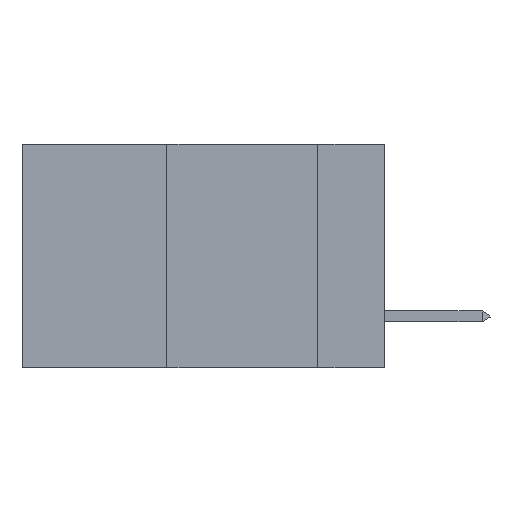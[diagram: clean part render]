
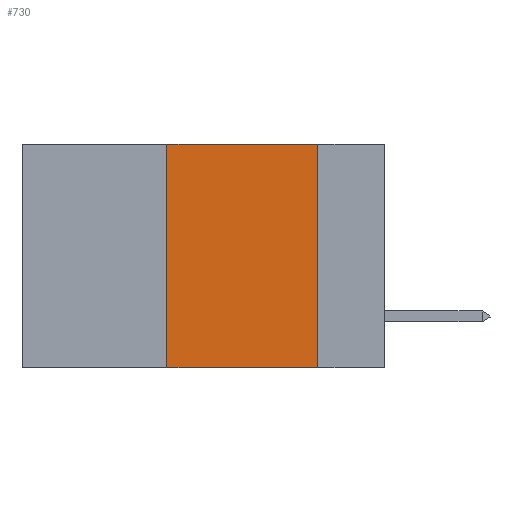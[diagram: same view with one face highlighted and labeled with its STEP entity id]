
A CAD part, left-side view. The second image highlights one B-rep face of the part: STEP entity #730.
In plain terms, the highlighted planar face has unit normal (-1, 0, 0).
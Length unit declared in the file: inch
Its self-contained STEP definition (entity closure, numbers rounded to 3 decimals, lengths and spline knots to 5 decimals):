
#730 = ADVANCED_FACE ( 'NONE', ( #17692 ), #5959, .F. ) ;
#867 = CARTESIAN_POINT ( 'NONE',  ( 0., 0.36, 0. ) ) ;
#1354 = CARTESIAN_POINT ( 'NONE',  ( 0., 0.11, 0. ) ) ;
#2589 = CARTESIAN_POINT ( 'NONE',  ( 0., 0.6, 0. ) ) ;
#3507 = LINE ( 'NONE', #2589, #7528 ) ;
#4113 = DIRECTION ( 'NONE',  ( 1., 0., 0. ) ) ;
#4148 = DIRECTION ( 'NONE',  ( 0., 0., -1. ) ) ;
#4427 = ORIENTED_EDGE ( 'NONE', *, *, #15269, .F. ) ;
#4691 = ORIENTED_EDGE ( 'NONE', *, *, #8674, .F. ) ;
#4712 = ORIENTED_EDGE ( 'NONE', *, *, #16273, .F. ) ;
#4762 = CARTESIAN_POINT ( 'NONE',  ( 0., 0.6, 0. ) ) ;
#4806 = ORIENTED_EDGE ( 'NONE', *, *, #5733, .T. ) ;
#5147 = VERTEX_POINT ( 'NONE', #1354 ) ;
#5433 = EDGE_LOOP ( 'NONE', ( #4427, #4712, #4691, #4806 ) ) ;
#5733 = EDGE_CURVE ( 'NONE', #13157, #16876, #14689, .T. ) ;
#5959 = PLANE ( 'NONE',  #11871 ) ;
#7170 = CARTESIAN_POINT ( 'NONE',  ( 0., 0.6, -0.37 ) ) ;
#7246 = LINE ( 'NONE', #867, #14372 ) ;
#7343 = LINE ( 'NONE', #16596, #14467 ) ;
#7528 = VECTOR ( 'NONE', #18067, 39.37008 ) ;
#8674 = EDGE_CURVE ( 'NONE', #13157, #15586, #7246, .T. ) ;
#10566 = DIRECTION ( 'NONE',  ( 0., -1., 0. ) ) ;
#11217 = DIRECTION ( 'NONE',  ( 0., 0., -1. ) ) ;
#11871 = AXIS2_PLACEMENT_3D ( 'NONE', #4762, #4113, #4148 ) ;
#13157 = VERTEX_POINT ( 'NONE', #15795 ) ;
#14101 = CARTESIAN_POINT ( 'NONE',  ( 0., 0.11, -0.37 ) ) ;
#14372 = VECTOR ( 'NONE', #17823, 39.37008 ) ;
#14467 = VECTOR ( 'NONE', #11217, 39.37008 ) ;
#14689 = LINE ( 'NONE', #7170, #17688 ) ;
#15269 = EDGE_CURVE ( 'NONE', #5147, #16876, #7343, .T. ) ;
#15586 = VERTEX_POINT ( 'NONE', #17879 ) ;
#15795 = CARTESIAN_POINT ( 'NONE',  ( 0., 0.36, -0.37 ) ) ;
#16273 = EDGE_CURVE ( 'NONE', #15586, #5147, #3507, .T. ) ;
#16596 = CARTESIAN_POINT ( 'NONE',  ( 0., 0.11, 0. ) ) ;
#16876 = VERTEX_POINT ( 'NONE', #14101 ) ;
#17688 = VECTOR ( 'NONE', #10566, 39.37008 ) ;
#17692 = FACE_OUTER_BOUND ( 'NONE', #5433, .T. ) ;
#17823 = DIRECTION ( 'NONE',  ( 0., 0., 1. ) ) ;
#17879 = CARTESIAN_POINT ( 'NONE',  ( 0., 0.36, 0. ) ) ;
#18067 = DIRECTION ( 'NONE',  ( 0., -1., 0. ) ) ;
